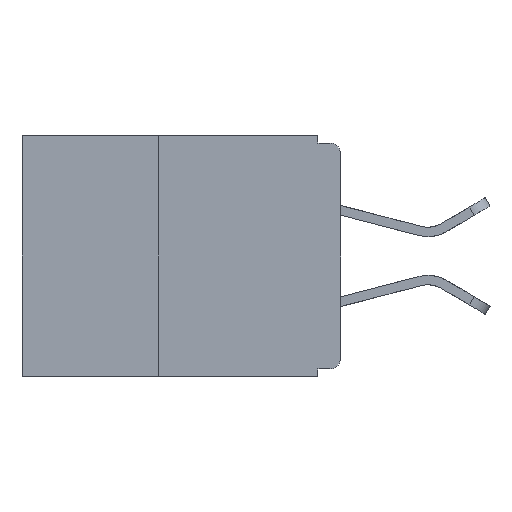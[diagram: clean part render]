
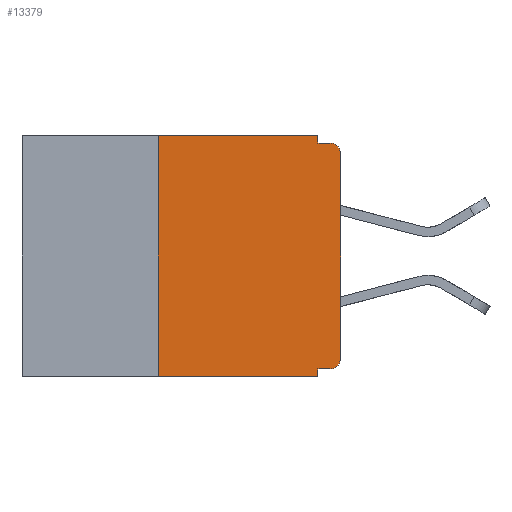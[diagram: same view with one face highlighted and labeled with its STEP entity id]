
A CAD part, left-side view. The second image highlights one B-rep face of the part: STEP entity #13379.
In plain terms, the highlighted planar face has unit normal (-1, 0, 0).
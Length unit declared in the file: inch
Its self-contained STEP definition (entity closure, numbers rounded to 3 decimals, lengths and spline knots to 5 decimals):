
#3 = DIRECTION ( 'NONE',  ( 0., 0., -1. ) ) ;
#531 = DIRECTION ( 'NONE',  ( 0., -1., 0. ) ) ;
#653 = DIRECTION ( 'NONE',  ( -1., 0., 0. ) ) ;
#865 = VECTOR ( 'NONE', #6977, 39.37008 ) ;
#1069 = ORIENTED_EDGE ( 'NONE', *, *, #13675, .F. ) ;
#1174 = VERTEX_POINT ( 'NONE', #1652 ) ;
#1355 = LINE ( 'NONE', #10129, #865 ) ;
#1603 = LINE ( 'NONE', #1971, #9557 ) ;
#1652 = CARTESIAN_POINT ( 'NONE',  ( 0., 0.25, -0.33 ) ) ;
#1971 = CARTESIAN_POINT ( 'NONE',  ( 0., 0.437, -0.33 ) ) ;
#2514 = CARTESIAN_POINT ( 'NONE',  ( 0., 0.437, 0. ) ) ;
#3574 = DIRECTION ( 'NONE',  ( 0., -1., 0. ) ) ;
#3692 = VECTOR ( 'NONE', #531, 39.37008 ) ;
#3874 = ORIENTED_EDGE ( 'NONE', *, *, #13589, .F. ) ;
#3892 = DIRECTION ( 'NONE',  ( 0., 0., 1. ) ) ;
#3933 = ORIENTED_EDGE ( 'NONE', *, *, #8773, .T. ) ;
#4189 = LINE ( 'NONE', #19228, #3692 ) ;
#4227 = VERTEX_POINT ( 'NONE', #10728 ) ;
#4823 = CARTESIAN_POINT ( 'NONE',  ( 0., 0., -0.01 ) ) ;
#4873 = VECTOR ( 'NONE', #18733, 39.37008 ) ;
#4919 = DIRECTION ( 'NONE',  ( 0., 0., -1. ) ) ;
#5647 = DIRECTION ( 'NONE',  ( -1., 0., 0. ) ) ;
#5761 = VERTEX_POINT ( 'NONE', #16225 ) ;
#5773 = DIRECTION ( 'NONE',  ( 1., 0., 0. ) ) ;
#6009 = VECTOR ( 'NONE', #18144, 39.37008 ) ;
#6343 = CARTESIAN_POINT ( 'NONE',  ( 0., 0.031, 0. ) ) ;
#6363 = EDGE_CURVE ( 'NONE', #7302, #5761, #4189, .T. ) ;
#6977 = DIRECTION ( 'NONE',  ( 0., 1., 0. ) ) ;
#7302 = VERTEX_POINT ( 'NONE', #11169 ) ;
#7921 = CIRCLE ( 'NONE', #10785, 0.015 ) ;
#7992 = ORIENTED_EDGE ( 'NONE', *, *, #8091, .F. ) ;
#8091 = EDGE_CURVE ( 'NONE', #19141, #18446, #1355, .T. ) ;
#8148 = CARTESIAN_POINT ( 'NONE',  ( 0., 0.031, -0.33 ) ) ;
#8413 = ORIENTED_EDGE ( 'NONE', *, *, #12749, .T. ) ;
#8498 = LINE ( 'NONE', #6343, #16243 ) ;
#8773 = EDGE_CURVE ( 'NONE', #10470, #9290, #7921, .T. ) ;
#8784 = CIRCLE ( 'NONE', #19927, 0.015 ) ;
#9176 = EDGE_CURVE ( 'NONE', #4227, #9290, #17310, .T. ) ;
#9290 = VERTEX_POINT ( 'NONE', #12934 ) ;
#9299 = CARTESIAN_POINT ( 'NONE',  ( 0., 0., -0.305 ) ) ;
#9557 = VECTOR ( 'NONE', #3574, 39.37008 ) ;
#10129 = CARTESIAN_POINT ( 'NONE',  ( 0., 0., -0.32 ) ) ;
#10182 = CARTESIAN_POINT ( 'NONE',  ( 0., 0.015, -0.025 ) ) ;
#10217 = LINE ( 'NONE', #15084, #6009 ) ;
#10470 = VERTEX_POINT ( 'NONE', #18829 ) ;
#10728 = CARTESIAN_POINT ( 'NONE',  ( 0., 0.031, -0.01 ) ) ;
#10785 = AXIS2_PLACEMENT_3D ( 'NONE', #10182, #653, #11737 ) ;
#11169 = CARTESIAN_POINT ( 'NONE',  ( 0., 0.25, 0. ) ) ;
#11401 = FACE_OUTER_BOUND ( 'NONE', #18248, .T. ) ;
#11737 = DIRECTION ( 'NONE',  ( 0., 0., -1. ) ) ;
#11924 = EDGE_CURVE ( 'NONE', #19141, #18007, #8784, .T. ) ;
#12296 = CARTESIAN_POINT ( 'NONE',  ( 0., 0.031, -0.33 ) ) ;
#12424 = ORIENTED_EDGE ( 'NONE', *, *, #9176, .F. ) ;
#12749 = EDGE_CURVE ( 'NONE', #18007, #10470, #10217, .T. ) ;
#12777 = ORIENTED_EDGE ( 'NONE', *, *, #11924, .T. ) ;
#12934 = CARTESIAN_POINT ( 'NONE',  ( 0., 0.015, -0.01 ) ) ;
#13379 = ADVANCED_FACE ( 'NONE', ( #11401 ), #15131, .F. ) ;
#13544 = ORIENTED_EDGE ( 'NONE', *, *, #6363, .F. ) ;
#13589 = EDGE_CURVE ( 'NONE', #1174, #7302, #16223, .T. ) ;
#13675 = EDGE_CURVE ( 'NONE', #18446, #18394, #18323, .T. ) ;
#14230 = ORIENTED_EDGE ( 'NONE', *, *, #19237, .T. ) ;
#15003 = CARTESIAN_POINT ( 'NONE',  ( 0., 0.015, -0.305 ) ) ;
#15084 = CARTESIAN_POINT ( 'NONE',  ( 0., 0., 0. ) ) ;
#15131 = PLANE ( 'NONE',  #16666 ) ;
#15249 = VECTOR ( 'NONE', #3892, 39.37008 ) ;
#15365 = ORIENTED_EDGE ( 'NONE', *, *, #16183, .F. ) ;
#15536 = CARTESIAN_POINT ( 'NONE',  ( 0., 0.031, -0.32 ) ) ;
#16183 = EDGE_CURVE ( 'NONE', #5761, #4227, #8498, .T. ) ;
#16223 = LINE ( 'NONE', #18698, #15249 ) ;
#16225 = CARTESIAN_POINT ( 'NONE',  ( 0., 0.031, 0. ) ) ;
#16243 = VECTOR ( 'NONE', #3, 39.37008 ) ;
#16544 = DIRECTION ( 'NONE',  ( 0., 0., -1. ) ) ;
#16666 = AXIS2_PLACEMENT_3D ( 'NONE', #2514, #5773, #16671 ) ;
#16671 = DIRECTION ( 'NONE',  ( 0., 0., -1. ) ) ;
#17310 = LINE ( 'NONE', #4823, #4873 ) ;
#17863 = VECTOR ( 'NONE', #4919, 39.37008 ) ;
#18007 = VERTEX_POINT ( 'NONE', #9299 ) ;
#18144 = DIRECTION ( 'NONE',  ( 0., 0., 1. ) ) ;
#18248 = EDGE_LOOP ( 'NONE', ( #8413, #3933, #12424, #15365, #13544, #3874, #14230, #1069, #7992, #12777 ) ) ;
#18323 = LINE ( 'NONE', #8148, #17863 ) ;
#18394 = VERTEX_POINT ( 'NONE', #12296 ) ;
#18446 = VERTEX_POINT ( 'NONE', #15536 ) ;
#18698 = CARTESIAN_POINT ( 'NONE',  ( 0., 0.25, -0.33 ) ) ;
#18733 = DIRECTION ( 'NONE',  ( 0., -1., 0. ) ) ;
#18799 = CARTESIAN_POINT ( 'NONE',  ( 0., 0.015, -0.32 ) ) ;
#18829 = CARTESIAN_POINT ( 'NONE',  ( 0., 0., -0.025 ) ) ;
#19141 = VERTEX_POINT ( 'NONE', #18799 ) ;
#19228 = CARTESIAN_POINT ( 'NONE',  ( 0., 0.437, 0. ) ) ;
#19237 = EDGE_CURVE ( 'NONE', #1174, #18394, #1603, .T. ) ;
#19927 = AXIS2_PLACEMENT_3D ( 'NONE', #15003, #5647, #16544 ) ;
